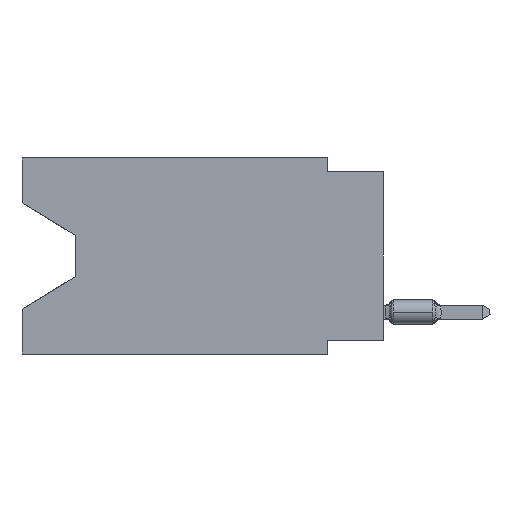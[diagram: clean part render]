
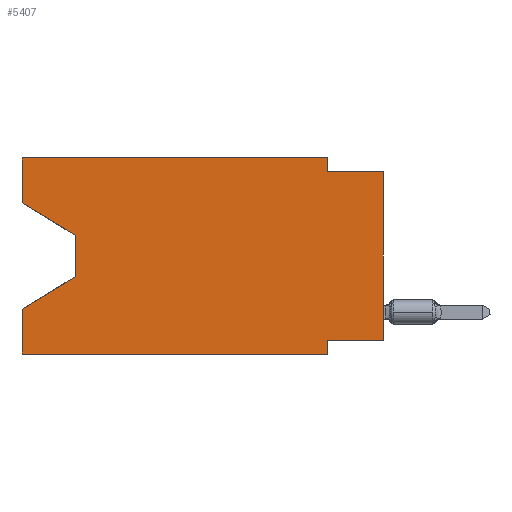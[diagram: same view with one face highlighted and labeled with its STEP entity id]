
A CAD part, left-side view. The second image highlights one B-rep face of the part: STEP entity #5407.
In plain terms, the highlighted planar face has unit normal (-1, 0, 0).
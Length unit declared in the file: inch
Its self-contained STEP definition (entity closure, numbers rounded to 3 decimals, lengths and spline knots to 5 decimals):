
#5 = DIRECTION ( 'NONE',  ( 0., 0.855, -0.519 ) ) ;
#8 = EDGE_CURVE ( 'NONE', #5666, #6866, #3084, .T. ) ;
#484 = DIRECTION ( 'NONE',  ( 0., 0., -1. ) ) ;
#491 = CARTESIAN_POINT ( 'NONE',  ( 0., 0., -0.025 ) ) ;
#557 = VECTOR ( 'NONE', #1482, 39.37008 ) ;
#920 = CARTESIAN_POINT ( 'NONE',  ( 0., 0.1, 0. ) ) ;
#993 = VERTEX_POINT ( 'NONE', #30597 ) ;
#1059 = CARTESIAN_POINT ( 'NONE',  ( 0., 0.645, 0. ) ) ;
#1140 = LINE ( 'NONE', #21092, #2375 ) ;
#1416 = CARTESIAN_POINT ( 'NONE',  ( 0., 0.645, -0.35 ) ) ;
#1482 = DIRECTION ( 'NONE',  ( 0., -0.855, -0.519 ) ) ;
#1667 = CARTESIAN_POINT ( 'NONE',  ( 0., 0.645, 0. ) ) ;
#1907 = VERTEX_POINT ( 'NONE', #23724 ) ;
#1931 = ORIENTED_EDGE ( 'NONE', *, *, #2639, .T. ) ;
#1932 = VERTEX_POINT ( 'NONE', #23562 ) ;
#2027 = CARTESIAN_POINT ( 'NONE',  ( 0., 0.55, -0.138 ) ) ;
#2256 = CARTESIAN_POINT ( 'NONE',  ( 0., 0.1, -0.325 ) ) ;
#2375 = VECTOR ( 'NONE', #25800, 39.37008 ) ;
#2639 = EDGE_CURVE ( 'NONE', #16316, #993, #15084, .T. ) ;
#3016 = DIRECTION ( 'NONE',  ( 0., -1., 0. ) ) ;
#3084 = LINE ( 'NONE', #9890, #21980 ) ;
#3266 = EDGE_CURVE ( 'NONE', #1907, #6866, #28471, .T. ) ;
#3538 = DIRECTION ( 'NONE',  ( 0., 0., 1. ) ) ;
#3672 = DIRECTION ( 'NONE',  ( 0., 0., -1. ) ) ;
#5407 = ADVANCED_FACE ( 'NONE', ( #6325 ), #6011, .F. ) ;
#5502 = LINE ( 'NONE', #30126, #6248 ) ;
#5666 = VERTEX_POINT ( 'NONE', #2256 ) ;
#6011 = PLANE ( 'NONE',  #26614 ) ;
#6248 = VECTOR ( 'NONE', #3538, 39.37008 ) ;
#6325 = FACE_OUTER_BOUND ( 'NONE', #31008, .T. ) ;
#6392 = VECTOR ( 'NONE', #3016, 39.37008 ) ;
#6581 = DIRECTION ( 'NONE',  ( 0., 0., 1. ) ) ;
#6673 = CARTESIAN_POINT ( 'NONE',  ( 0., 0., -0.325 ) ) ;
#6866 = VERTEX_POINT ( 'NONE', #22385 ) ;
#7074 = CARTESIAN_POINT ( 'NONE',  ( 0., 0.1, 0. ) ) ;
#7079 = VERTEX_POINT ( 'NONE', #491 ) ;
#7208 = ORIENTED_EDGE ( 'NONE', *, *, #16284, .F. ) ;
#7966 = VECTOR ( 'NONE', #17055, 39.37008 ) ;
#8766 = LINE ( 'NONE', #19155, #557 ) ;
#9233 = VERTEX_POINT ( 'NONE', #6673 ) ;
#9283 = CARTESIAN_POINT ( 'NONE',  ( 0., 0.55, -0.212 ) ) ;
#9717 = LINE ( 'NONE', #26745, #10391 ) ;
#9890 = CARTESIAN_POINT ( 'NONE',  ( 0., 0.1, -0.35 ) ) ;
#10274 = CARTESIAN_POINT ( 'NONE',  ( 0., 0.1, -0.025 ) ) ;
#10391 = VECTOR ( 'NONE', #19768, 39.37008 ) ;
#11192 = DIRECTION ( 'NONE',  ( 1., 0., 0. ) ) ;
#11314 = EDGE_CURVE ( 'NONE', #24103, #1932, #21329, .T. ) ;
#11990 = CARTESIAN_POINT ( 'NONE',  ( 0., 0.55, -0.212 ) ) ;
#12608 = VECTOR ( 'NONE', #5, 39.37008 ) ;
#12630 = ORIENTED_EDGE ( 'NONE', *, *, #11314, .F. ) ;
#13342 = ORIENTED_EDGE ( 'NONE', *, *, #25397, .T. ) ;
#13384 = ORIENTED_EDGE ( 'NONE', *, *, #3266, .T. ) ;
#13429 = VERTEX_POINT ( 'NONE', #10274 ) ;
#13881 = EDGE_CURVE ( 'NONE', #9233, #5666, #1140, .T. ) ;
#14229 = LINE ( 'NONE', #31245, #15254 ) ;
#15084 = LINE ( 'NONE', #11990, #12608 ) ;
#15254 = VECTOR ( 'NONE', #16346, 39.37008 ) ;
#15581 = CARTESIAN_POINT ( 'NONE',  ( 0., 0.645, -0.08025 ) ) ;
#16284 = EDGE_CURVE ( 'NONE', #1932, #20358, #21763, .T. ) ;
#16316 = VERTEX_POINT ( 'NONE', #9283 ) ;
#16346 = DIRECTION ( 'NONE',  ( 0., 0., 1. ) ) ;
#17055 = DIRECTION ( 'NONE',  ( 0., -1., 0. ) ) ;
#17110 = EDGE_CURVE ( 'NONE', #1907, #993, #14229, .T. ) ;
#19155 = CARTESIAN_POINT ( 'NONE',  ( 0., 0.645, -0.08025 ) ) ;
#19572 = LINE ( 'NONE', #25228, #6392 ) ;
#19768 = DIRECTION ( 'NONE',  ( 0., 0., -1. ) ) ;
#20358 = VERTEX_POINT ( 'NONE', #7074 ) ;
#20543 = EDGE_CURVE ( 'NONE', #13429, #7079, #19572, .T. ) ;
#21092 = CARTESIAN_POINT ( 'NONE',  ( 0., 0., -0.325 ) ) ;
#21183 = DIRECTION ( 'NONE',  ( 0., -1., 0. ) ) ;
#21329 = LINE ( 'NONE', #1059, #31419 ) ;
#21763 = LINE ( 'NONE', #1667, #7966 ) ;
#21980 = VECTOR ( 'NONE', #484, 39.37008 ) ;
#22385 = CARTESIAN_POINT ( 'NONE',  ( 0., 0.1, -0.35 ) ) ;
#22915 = EDGE_CURVE ( 'NONE', #23684, #16316, #9717, .T. ) ;
#23000 = EDGE_CURVE ( 'NONE', #9233, #7079, #5502, .T. ) ;
#23143 = LINE ( 'NONE', #920, #26502 ) ;
#23253 = ORIENTED_EDGE ( 'NONE', *, *, #27232, .F. ) ;
#23562 = CARTESIAN_POINT ( 'NONE',  ( 0., 0.645, 0. ) ) ;
#23684 = VERTEX_POINT ( 'NONE', #2027 ) ;
#23724 = CARTESIAN_POINT ( 'NONE',  ( 0., 0.645, -0.35 ) ) ;
#24103 = VERTEX_POINT ( 'NONE', #15581 ) ;
#24679 = ORIENTED_EDGE ( 'NONE', *, *, #23000, .T. ) ;
#25092 = ORIENTED_EDGE ( 'NONE', *, *, #22915, .T. ) ;
#25228 = CARTESIAN_POINT ( 'NONE',  ( 0., 0., -0.025 ) ) ;
#25397 = EDGE_CURVE ( 'NONE', #24103, #23684, #8766, .T. ) ;
#25800 = DIRECTION ( 'NONE',  ( 0., 1., 0. ) ) ;
#26502 = VECTOR ( 'NONE', #3672, 39.37008 ) ;
#26614 = AXIS2_PLACEMENT_3D ( 'NONE', #28528, #11192, #30645 ) ;
#26745 = CARTESIAN_POINT ( 'NONE',  ( 0., 0.55, -0.138 ) ) ;
#26839 = ORIENTED_EDGE ( 'NONE', *, *, #8, .F. ) ;
#27232 = EDGE_CURVE ( 'NONE', #20358, #13429, #23143, .T. ) ;
#28170 = VECTOR ( 'NONE', #21183, 39.37008 ) ;
#28471 = LINE ( 'NONE', #1416, #28170 ) ;
#28528 = CARTESIAN_POINT ( 'NONE',  ( 0., 0.645, 0. ) ) ;
#29052 = ORIENTED_EDGE ( 'NONE', *, *, #13881, .F. ) ;
#30126 = CARTESIAN_POINT ( 'NONE',  ( 0., 0., 0. ) ) ;
#30321 = ORIENTED_EDGE ( 'NONE', *, *, #20543, .F. ) ;
#30597 = CARTESIAN_POINT ( 'NONE',  ( 0., 0.645, -0.26975 ) ) ;
#30645 = DIRECTION ( 'NONE',  ( 0., 0., -1. ) ) ;
#31008 = EDGE_LOOP ( 'NONE', ( #13342, #25092, #1931, #31512, #13384, #26839, #29052, #24679, #30321, #23253, #7208, #12630 ) ) ;
#31245 = CARTESIAN_POINT ( 'NONE',  ( 0., 0.645, 0. ) ) ;
#31419 = VECTOR ( 'NONE', #6581, 39.37008 ) ;
#31512 = ORIENTED_EDGE ( 'NONE', *, *, #17110, .F. ) ;
